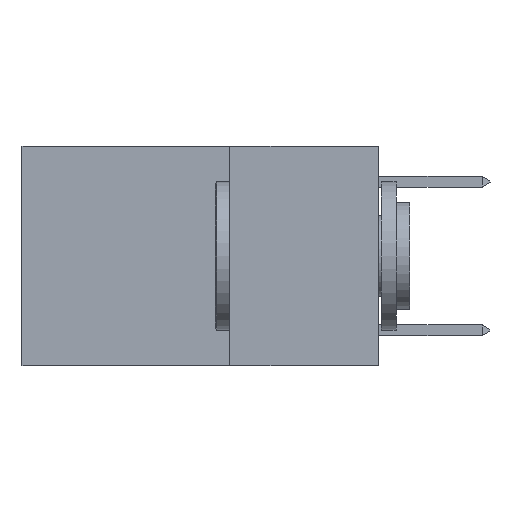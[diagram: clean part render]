
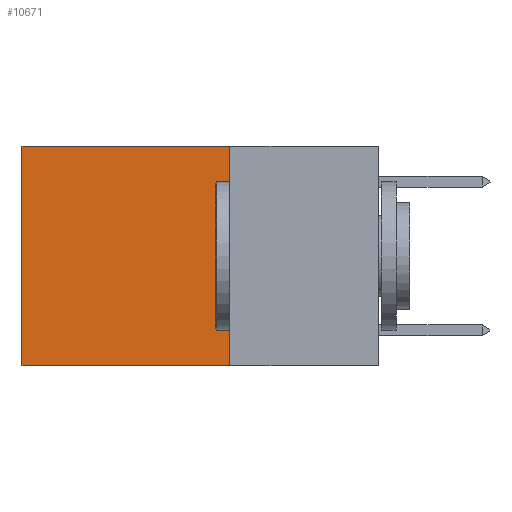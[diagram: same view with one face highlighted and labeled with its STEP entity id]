
A CAD part, left-side view. The second image highlights one B-rep face of the part: STEP entity #10671.
In plain terms, the highlighted planar face has unit normal (-1, 0, 0).
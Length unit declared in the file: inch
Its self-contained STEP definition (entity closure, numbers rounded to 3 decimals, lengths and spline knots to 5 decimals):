
#311 = ORIENTED_EDGE ( 'NONE', *, *, #4856, .T. ) ;
#326 = VERTEX_POINT ( 'NONE', #5299 ) ;
#405 = ORIENTED_EDGE ( 'NONE', *, *, #5873, .F. ) ;
#670 = ORIENTED_EDGE ( 'NONE', *, *, #7594, .F. ) ;
#730 = DIRECTION ( 'NONE',  ( 0., 1., 0. ) ) ;
#1000 = DIRECTION ( 'NONE',  ( 0., 0., -1. ) ) ;
#1374 = VECTOR ( 'NONE', #9322, 39.37008 ) ;
#1689 = VECTOR ( 'NONE', #1000, 39.37008 ) ;
#1920 = LINE ( 'NONE', #4886, #9114 ) ;
#3377 = EDGE_LOOP ( 'NONE', ( #311, #670, #405, #12104 ) ) ;
#4227 = LINE ( 'NONE', #12037, #1689 ) ;
#4257 = CARTESIAN_POINT ( 'NONE',  ( 0.2625, 0.6, 0. ) ) ;
#4856 = EDGE_CURVE ( 'NONE', #9137, #7884, #4227, .T. ) ;
#4886 = CARTESIAN_POINT ( 'NONE',  ( 0.2625, 0.25, 0. ) ) ;
#5211 = DIRECTION ( 'NONE',  ( 1., 0., 0. ) ) ;
#5299 = CARTESIAN_POINT ( 'NONE',  ( 0.2625, 0.25, -0.37 ) ) ;
#5335 = LINE ( 'NONE', #7403, #1374 ) ;
#5873 = EDGE_CURVE ( 'NONE', #9845, #326, #5335, .T. ) ;
#6904 = LINE ( 'NONE', #10658, #11779 ) ;
#7403 = CARTESIAN_POINT ( 'NONE',  ( 0.2625, 0.25, 0. ) ) ;
#7594 = EDGE_CURVE ( 'NONE', #326, #7884, #6904, .T. ) ;
#7884 = VERTEX_POINT ( 'NONE', #12919 ) ;
#8513 = PLANE ( 'NONE',  #9134 ) ;
#8973 = DIRECTION ( 'NONE',  ( 0., 1., 0. ) ) ;
#9114 = VECTOR ( 'NONE', #8973, 39.37008 ) ;
#9134 = AXIS2_PLACEMENT_3D ( 'NONE', #10242, #5211, #9243 ) ;
#9137 = VERTEX_POINT ( 'NONE', #4257 ) ;
#9243 = DIRECTION ( 'NONE',  ( 0., 0., -1. ) ) ;
#9322 = DIRECTION ( 'NONE',  ( 0., 0., -1. ) ) ;
#9567 = EDGE_CURVE ( 'NONE', #9845, #9137, #1920, .T. ) ;
#9845 = VERTEX_POINT ( 'NONE', #10015 ) ;
#10015 = CARTESIAN_POINT ( 'NONE',  ( 0.2625, 0.25, 0. ) ) ;
#10242 = CARTESIAN_POINT ( 'NONE',  ( 0.2625, 0.25, 0. ) ) ;
#10658 = CARTESIAN_POINT ( 'NONE',  ( 0.2625, 0.25, -0.37 ) ) ;
#10671 = ADVANCED_FACE ( 'NONE', ( #11308 ), #8513, .F. ) ;
#11308 = FACE_OUTER_BOUND ( 'NONE', #3377, .T. ) ;
#11779 = VECTOR ( 'NONE', #730, 39.37008 ) ;
#12037 = CARTESIAN_POINT ( 'NONE',  ( 0.2625, 0.6, 0. ) ) ;
#12104 = ORIENTED_EDGE ( 'NONE', *, *, #9567, .T. ) ;
#12919 = CARTESIAN_POINT ( 'NONE',  ( 0.2625, 0.6, -0.37 ) ) ;
